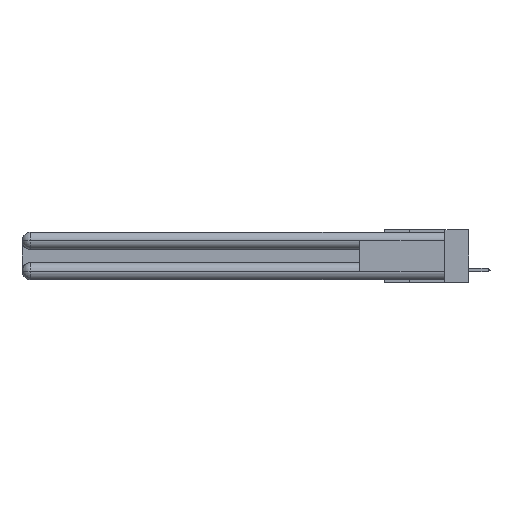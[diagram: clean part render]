
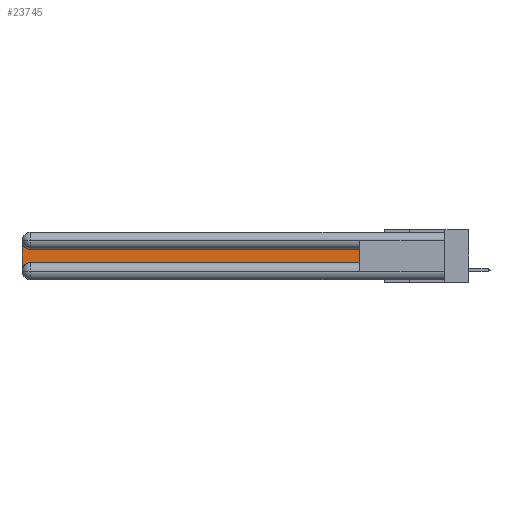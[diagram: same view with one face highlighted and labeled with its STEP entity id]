
A CAD part, left-side view. The second image highlights one B-rep face of the part: STEP entity #23745.
In plain terms, the highlighted planar face has unit normal (-1, 0, 0).
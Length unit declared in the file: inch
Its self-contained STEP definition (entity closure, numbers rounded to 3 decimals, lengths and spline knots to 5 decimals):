
#153 = EDGE_LOOP ( 'NONE', ( #5372, #24489, #5181, #12325, #14993, #16776 ) ) ;
#568 = CARTESIAN_POINT ( 'NONE',  ( 0.075, 3., -0.2775 ) ) ;
#2367 = DIRECTION ( 'NONE',  ( 0., 0., 1. ) ) ;
#2951 = VERTEX_POINT ( 'NONE', #25012 ) ;
#3377 = CARTESIAN_POINT ( 'NONE',  ( 0.075, 3., -0.0625 ) ) ;
#3959 = DIRECTION ( 'NONE',  ( 1., 0., 0. ) ) ;
#4219 = DIRECTION ( 'NONE',  ( 0., -1., 0. ) ) ;
#4413 = LINE ( 'NONE', #15863, #11522 ) ;
#5124 = EDGE_CURVE ( 'NONE', #23459, #20744, #4413, .T. ) ;
#5181 = ORIENTED_EDGE ( 'NONE', *, *, #5124, .T. ) ;
#5372 = ORIENTED_EDGE ( 'NONE', *, *, #21344, .T. ) ;
#7111 = EDGE_CURVE ( 'NONE', #20744, #10773, #21757, .T. ) ;
#8587 = CARTESIAN_POINT ( 'NONE',  ( 0.075, 0.6, -0.2175 ) ) ;
#8851 = VECTOR ( 'NONE', #2367, 39.37008 ) ;
#9108 = CARTESIAN_POINT ( 'NONE',  ( 0.075, 0.6, -0.1225 ) ) ;
#9622 = DIRECTION ( 'NONE',  ( 0., 0., -1. ) ) ;
#10769 = CARTESIAN_POINT ( 'NONE',  ( 0.075, 0.6, -0.2175 ) ) ;
#10773 = VERTEX_POINT ( 'NONE', #20800 ) ;
#11485 = VECTOR ( 'NONE', #11693, 39.37008 ) ;
#11522 = VECTOR ( 'NONE', #9622, 39.37008 ) ;
#11693 = DIRECTION ( 'NONE',  ( 0., 1., 0. ) ) ;
#12325 = ORIENTED_EDGE ( 'NONE', *, *, #7111, .T. ) ;
#12735 = DIRECTION ( 'NONE',  ( 0., 0., -1. ) ) ;
#12841 = PLANE ( 'NONE',  #13820 ) ;
#13551 = LINE ( 'NONE', #8587, #8851 ) ;
#13820 = AXIS2_PLACEMENT_3D ( 'NONE', #23514, #26056, #19451 ) ;
#14120 = AXIS2_PLACEMENT_3D ( 'NONE', #25495, #3959, #12735 ) ;
#14172 = DIRECTION ( 'NONE',  ( 0., 0., -1. ) ) ;
#14993 = ORIENTED_EDGE ( 'NONE', *, *, #26114, .T. ) ;
#15863 = CARTESIAN_POINT ( 'NONE',  ( 0.075, 3., -0.2175 ) ) ;
#16234 = CARTESIAN_POINT ( 'NONE',  ( 0.075, 2.94, -0.0625 ) ) ;
#16776 = ORIENTED_EDGE ( 'NONE', *, *, #20832, .T. ) ;
#17466 = AXIS2_PLACEMENT_3D ( 'NONE', #16234, #27045, #14172 ) ;
#19451 = DIRECTION ( 'NONE',  ( 0., 0., -1. ) ) ;
#20744 = VERTEX_POINT ( 'NONE', #568 ) ;
#20800 = CARTESIAN_POINT ( 'NONE',  ( 0.075, 2.94, -0.2175 ) ) ;
#20832 = EDGE_CURVE ( 'NONE', #27487, #21821, #13551, .T. ) ;
#21000 = VECTOR ( 'NONE', #4219, 39.37008 ) ;
#21344 = EDGE_CURVE ( 'NONE', #21821, #2951, #26266, .T. ) ;
#21757 = CIRCLE ( 'NONE', #14120, 0.06 ) ;
#21821 = VERTEX_POINT ( 'NONE', #9108 ) ;
#22351 = LINE ( 'NONE', #10769, #21000 ) ;
#22946 = CIRCLE ( 'NONE', #17466, 0.06 ) ;
#23459 = VERTEX_POINT ( 'NONE', #3377 ) ;
#23514 = CARTESIAN_POINT ( 'NONE',  ( 0.075, 3., -0.1225 ) ) ;
#23745 = ADVANCED_FACE ( 'NONE', ( #26533 ), #12841, .F. ) ;
#24489 = ORIENTED_EDGE ( 'NONE', *, *, #27217, .T. ) ;
#24553 = CARTESIAN_POINT ( 'NONE',  ( 0.075, 0.6, -0.1225 ) ) ;
#25012 = CARTESIAN_POINT ( 'NONE',  ( 0.075, 2.94, -0.1225 ) ) ;
#25495 = CARTESIAN_POINT ( 'NONE',  ( 0.075, 2.94, -0.2775 ) ) ;
#25645 = CARTESIAN_POINT ( 'NONE',  ( 0.075, 0.6, -0.2175 ) ) ;
#26056 = DIRECTION ( 'NONE',  ( 1., 0., 0. ) ) ;
#26114 = EDGE_CURVE ( 'NONE', #10773, #27487, #22351, .T. ) ;
#26266 = LINE ( 'NONE', #24553, #11485 ) ;
#26533 = FACE_OUTER_BOUND ( 'NONE', #153, .T. ) ;
#27045 = DIRECTION ( 'NONE',  ( 1., 0., 0. ) ) ;
#27217 = EDGE_CURVE ( 'NONE', #2951, #23459, #22946, .T. ) ;
#27487 = VERTEX_POINT ( 'NONE', #25645 ) ;
